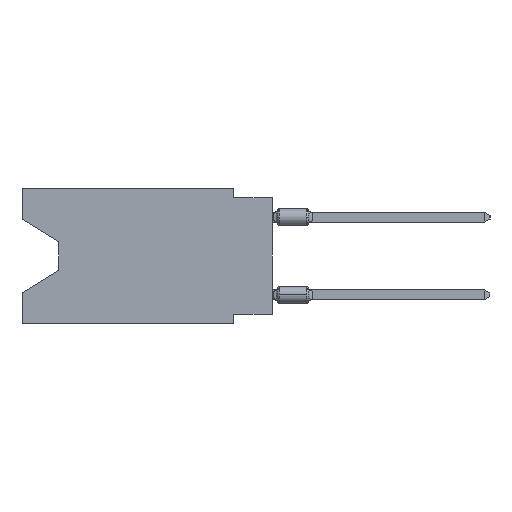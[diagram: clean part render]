
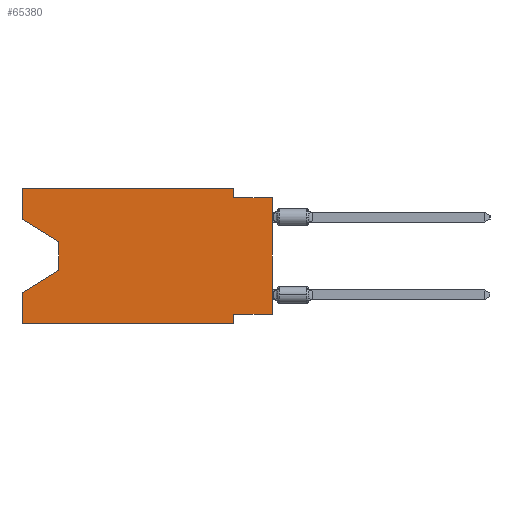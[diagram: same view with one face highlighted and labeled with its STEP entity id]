
A CAD part, left-side view. The second image highlights one B-rep face of the part: STEP entity #65380.
In plain terms, the highlighted planar face has unit normal (-1, 0, 0).
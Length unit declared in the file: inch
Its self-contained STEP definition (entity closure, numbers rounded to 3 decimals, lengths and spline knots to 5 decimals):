
#93 = CARTESIAN_POINT ( 'NONE',  ( 0., 0.1, -0.025 ) ) ;
#662 = ORIENTED_EDGE ( 'NONE', *, *, #49950, .T. ) ;
#2258 = ORIENTED_EDGE ( 'NONE', *, *, #20693, .F. ) ;
#2414 = VECTOR ( 'NONE', #8458, 39.37008 ) ;
#2709 = ORIENTED_EDGE ( 'NONE', *, *, #32529, .F. ) ;
#3036 = VECTOR ( 'NONE', #25514, 39.37008 ) ;
#3092 = CARTESIAN_POINT ( 'NONE',  ( 0., 0.1, -0.35 ) ) ;
#3550 = VECTOR ( 'NONE', #16048, 39.37008 ) ;
#4203 = ORIENTED_EDGE ( 'NONE', *, *, #51855, .F. ) ;
#4302 = LINE ( 'NONE', #19911, #27249 ) ;
#4640 = DIRECTION ( 'NONE',  ( 0., 0.855, -0.519 ) ) ;
#5428 = ORIENTED_EDGE ( 'NONE', *, *, #13291, .F. ) ;
#6548 = DIRECTION ( 'NONE',  ( 1., 0., 0. ) ) ;
#7391 = VERTEX_POINT ( 'NONE', #48860 ) ;
#7684 = DIRECTION ( 'NONE',  ( 0., 0., -1. ) ) ;
#8458 = DIRECTION ( 'NONE',  ( 0., -1., 0. ) ) ;
#10139 = ORIENTED_EDGE ( 'NONE', *, *, #16433, .T. ) ;
#10294 = VERTEX_POINT ( 'NONE', #45222 ) ;
#10690 = CARTESIAN_POINT ( 'NONE',  ( 0., 0., -0.025 ) ) ;
#10939 = VERTEX_POINT ( 'NONE', #27456 ) ;
#11841 = CARTESIAN_POINT ( 'NONE',  ( 0., 0.645, 0. ) ) ;
#11873 = VECTOR ( 'NONE', #55779, 39.37008 ) ;
#12184 = VERTEX_POINT ( 'NONE', #36570 ) ;
#12337 = DIRECTION ( 'NONE',  ( 0., -1., 0. ) ) ;
#13291 = EDGE_CURVE ( 'NONE', #18950, #51292, #13415, .T. ) ;
#13415 = LINE ( 'NONE', #49712, #48471 ) ;
#13846 = LINE ( 'NONE', #39801, #25340 ) ;
#14942 = DIRECTION ( 'NONE',  ( 0., -0.855, -0.519 ) ) ;
#16048 = DIRECTION ( 'NONE',  ( 0., -1., 0. ) ) ;
#16144 = EDGE_LOOP ( 'NONE', ( #45794, #662, #52000, #5428, #27194, #2709, #26498, #10139, #4203, #21161, #50932, #2258 ) ) ;
#16433 = EDGE_CURVE ( 'NONE', #10939, #34046, #4302, .T. ) ;
#16947 = VECTOR ( 'NONE', #12337, 39.37008 ) ;
#17352 = LINE ( 'NONE', #42992, #3550 ) ;
#18942 = LINE ( 'NONE', #55219, #40732 ) ;
#18950 = VERTEX_POINT ( 'NONE', #51904 ) ;
#19529 = VERTEX_POINT ( 'NONE', #93 ) ;
#19911 = CARTESIAN_POINT ( 'NONE',  ( 0., 0., 0. ) ) ;
#20693 = EDGE_CURVE ( 'NONE', #59464, #7391, #13846, .T. ) ;
#21161 = ORIENTED_EDGE ( 'NONE', *, *, #51905, .F. ) ;
#22376 = EDGE_CURVE ( 'NONE', #59464, #54222, #44917, .T. ) ;
#22481 = DIRECTION ( 'NONE',  ( 0., 0., -1. ) ) ;
#23345 = DIRECTION ( 'NONE',  ( 0., 0., -1. ) ) ;
#24812 = CARTESIAN_POINT ( 'NONE',  ( 0., 0., -0.325 ) ) ;
#25340 = VECTOR ( 'NONE', #34502, 39.37008 ) ;
#25514 = DIRECTION ( 'NONE',  ( 0., 0., -1. ) ) ;
#26498 = ORIENTED_EDGE ( 'NONE', *, *, #42872, .F. ) ;
#27194 = ORIENTED_EDGE ( 'NONE', *, *, #62178, .T. ) ;
#27249 = VECTOR ( 'NONE', #55208, 39.37008 ) ;
#27456 = CARTESIAN_POINT ( 'NONE',  ( 0., 0., -0.325 ) ) ;
#27511 = PLANE ( 'NONE',  #61029 ) ;
#30703 = EDGE_CURVE ( 'NONE', #37345, #51292, #18942, .T. ) ;
#32529 = EDGE_CURVE ( 'NONE', #12184, #10294, #57644, .T. ) ;
#33429 = LINE ( 'NONE', #60047, #2414 ) ;
#34046 = VERTEX_POINT ( 'NONE', #38093 ) ;
#34502 = DIRECTION ( 'NONE',  ( 0., 0., 1. ) ) ;
#36148 = VECTOR ( 'NONE', #14942, 39.37008 ) ;
#36490 = CARTESIAN_POINT ( 'NONE',  ( 0., 0.645, -0.26975 ) ) ;
#36570 = CARTESIAN_POINT ( 'NONE',  ( 0., 0.1, -0.325 ) ) ;
#37286 = CARTESIAN_POINT ( 'NONE',  ( 0., 0.1, 0. ) ) ;
#37345 = VERTEX_POINT ( 'NONE', #62154 ) ;
#38093 = CARTESIAN_POINT ( 'NONE',  ( 0., 0., -0.025 ) ) ;
#39801 = CARTESIAN_POINT ( 'NONE',  ( 0., 0.645, 0. ) ) ;
#40732 = VECTOR ( 'NONE', #4640, 39.37008 ) ;
#41448 = CARTESIAN_POINT ( 'NONE',  ( 0., 0.55, -0.138 ) ) ;
#42134 = LINE ( 'NONE', #41448, #3036 ) ;
#42872 = EDGE_CURVE ( 'NONE', #10939, #12184, #60118, .T. ) ;
#42992 = CARTESIAN_POINT ( 'NONE',  ( 0., 0.645, -0.35 ) ) ;
#43371 = DIRECTION ( 'NONE',  ( 0., 0., 1. ) ) ;
#44917 = LINE ( 'NONE', #45894, #36148 ) ;
#45222 = CARTESIAN_POINT ( 'NONE',  ( 0., 0.1, -0.35 ) ) ;
#45794 = ORIENTED_EDGE ( 'NONE', *, *, #22376, .T. ) ;
#45894 = CARTESIAN_POINT ( 'NONE',  ( 0., 0.645, -0.08025 ) ) ;
#47806 = VECTOR ( 'NONE', #7684, 39.37008 ) ;
#48471 = VECTOR ( 'NONE', #43371, 39.37008 ) ;
#48669 = VERTEX_POINT ( 'NONE', #52473 ) ;
#48860 = CARTESIAN_POINT ( 'NONE',  ( 0., 0.645, 0. ) ) ;
#49712 = CARTESIAN_POINT ( 'NONE',  ( 0., 0.645, 0. ) ) ;
#49950 = EDGE_CURVE ( 'NONE', #54222, #37345, #42134, .T. ) ;
#50085 = CARTESIAN_POINT ( 'NONE',  ( 0., 0.55, -0.138 ) ) ;
#50932 = ORIENTED_EDGE ( 'NONE', *, *, #63101, .F. ) ;
#51292 = VERTEX_POINT ( 'NONE', #36490 ) ;
#51855 = EDGE_CURVE ( 'NONE', #19529, #34046, #56308, .T. ) ;
#51904 = CARTESIAN_POINT ( 'NONE',  ( 0., 0.645, -0.35 ) ) ;
#51905 = EDGE_CURVE ( 'NONE', #48669, #19529, #53286, .T. ) ;
#52000 = ORIENTED_EDGE ( 'NONE', *, *, #30703, .T. ) ;
#52473 = CARTESIAN_POINT ( 'NONE',  ( 0., 0.1, 0. ) ) ;
#52828 = FACE_OUTER_BOUND ( 'NONE', #16144, .T. ) ;
#53286 = LINE ( 'NONE', #37286, #47806 ) ;
#54222 = VERTEX_POINT ( 'NONE', #50085 ) ;
#55208 = DIRECTION ( 'NONE',  ( 0., 0., 1. ) ) ;
#55219 = CARTESIAN_POINT ( 'NONE',  ( 0., 0.55, -0.212 ) ) ;
#55453 = CARTESIAN_POINT ( 'NONE',  ( 0., 0.645, -0.08025 ) ) ;
#55779 = DIRECTION ( 'NONE',  ( 0., 1., 0. ) ) ;
#56308 = LINE ( 'NONE', #10690, #16947 ) ;
#56943 = VECTOR ( 'NONE', #23345, 39.37008 ) ;
#57644 = LINE ( 'NONE', #3092, #56943 ) ;
#59464 = VERTEX_POINT ( 'NONE', #55453 ) ;
#60047 = CARTESIAN_POINT ( 'NONE',  ( 0., 0.645, 0. ) ) ;
#60118 = LINE ( 'NONE', #24812, #11873 ) ;
#61029 = AXIS2_PLACEMENT_3D ( 'NONE', #11841, #6548, #22481 ) ;
#62154 = CARTESIAN_POINT ( 'NONE',  ( 0., 0.55, -0.212 ) ) ;
#62178 = EDGE_CURVE ( 'NONE', #18950, #10294, #17352, .T. ) ;
#63101 = EDGE_CURVE ( 'NONE', #7391, #48669, #33429, .T. ) ;
#65380 = ADVANCED_FACE ( 'NONE', ( #52828 ), #27511, .F. ) ;
